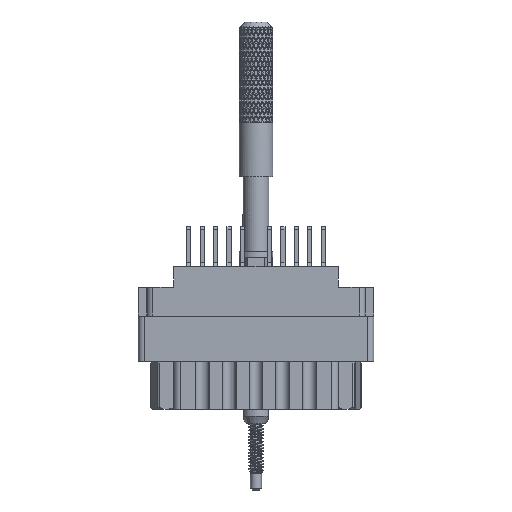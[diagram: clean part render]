
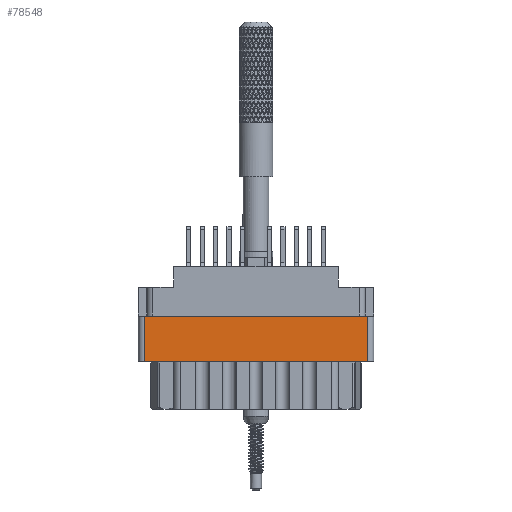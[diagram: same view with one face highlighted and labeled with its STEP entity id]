
A CAD part, front view. The second image highlights one B-rep face of the part: STEP entity #78548.
In plain terms, the highlighted planar face has unit normal (0, -1, 0).
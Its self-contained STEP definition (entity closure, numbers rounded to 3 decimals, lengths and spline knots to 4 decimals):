
#3311 = LINE ( 'NONE', #150773, #119535 ) ;
#8860 = CARTESIAN_POINT ( 'NONE',  ( -0.656, -0.343, -0.798 ) ) ;
#22287 = VERTEX_POINT ( 'NONE', #177488 ) ;
#29093 = VERTEX_POINT ( 'NONE', #193896 ) ;
#32149 = VECTOR ( 'NONE', #153689, 39.3701 ) ;
#37348 = ORIENTED_EDGE ( 'NONE', *, *, #55393, .T. ) ;
#53288 = PLANE ( 'NONE',  #153083 ) ;
#54508 = DIRECTION ( 'NONE',  ( -1., 0., 0. ) ) ;
#55393 = EDGE_CURVE ( 'NONE', #174596, #116888, #3311, .T. ) ;
#68156 = EDGE_CURVE ( 'NONE', #174596, #29093, #188779, .T. ) ;
#78548 = ADVANCED_FACE ( 'NONE', ( #183265 ), #53288, .T. ) ;
#78814 = EDGE_LOOP ( 'NONE', ( #173094, #37348, #144014, #162347 ) ) ;
#86216 = CARTESIAN_POINT ( 'NONE',  ( 0., -0.343, -0.529 ) ) ;
#89090 = DIRECTION ( 'NONE',  ( 0., 0., -1. ) ) ;
#98511 = EDGE_CURVE ( 'NONE', #22287, #116888, #161793, .T. ) ;
#106376 = LINE ( 'NONE', #111510, #149213 ) ;
#111510 = CARTESIAN_POINT ( 'NONE',  ( 0.624, -0.343, -0.798 ) ) ;
#116187 = DIRECTION ( 'NONE',  ( 0., 0., -1. ) ) ;
#116888 = VERTEX_POINT ( 'NONE', #164534 ) ;
#119535 = VECTOR ( 'NONE', #89090, 39.3701 ) ;
#144014 = ORIENTED_EDGE ( 'NONE', *, *, #98511, .F. ) ;
#144975 = CARTESIAN_POINT ( 'NONE',  ( -0.624, -0.343, -0.277 ) ) ;
#149213 = VECTOR ( 'NONE', #156636, 39.3701 ) ;
#150773 = CARTESIAN_POINT ( 'NONE',  ( -0.624, -0.343, -0.798 ) ) ;
#153083 = AXIS2_PLACEMENT_3D ( 'NONE', #8860, #191806, #116187 ) ;
#153689 = DIRECTION ( 'NONE',  ( 1., 0., 0. ) ) ;
#156636 = DIRECTION ( 'NONE',  ( 0., 0., 1. ) ) ;
#161793 = LINE ( 'NONE', #86216, #190582 ) ;
#162347 = ORIENTED_EDGE ( 'NONE', *, *, #162590, .T. ) ;
#162590 = EDGE_CURVE ( 'NONE', #22287, #29093, #106376, .T. ) ;
#164534 = CARTESIAN_POINT ( 'NONE',  ( -0.624, -0.343, -0.529 ) ) ;
#168309 = CARTESIAN_POINT ( 'NONE',  ( 0., -0.343, -0.277 ) ) ;
#173094 = ORIENTED_EDGE ( 'NONE', *, *, #68156, .F. ) ;
#174596 = VERTEX_POINT ( 'NONE', #144975 ) ;
#177488 = CARTESIAN_POINT ( 'NONE',  ( 0.624, -0.343, -0.529 ) ) ;
#183265 = FACE_OUTER_BOUND ( 'NONE', #78814, .T. ) ;
#188779 = LINE ( 'NONE', #168309, #32149 ) ;
#190582 = VECTOR ( 'NONE', #54508, 39.3701 ) ;
#191806 = DIRECTION ( 'NONE',  ( 0., -1., 0. ) ) ;
#193896 = CARTESIAN_POINT ( 'NONE',  ( 0.624, -0.343, -0.277 ) ) ;
